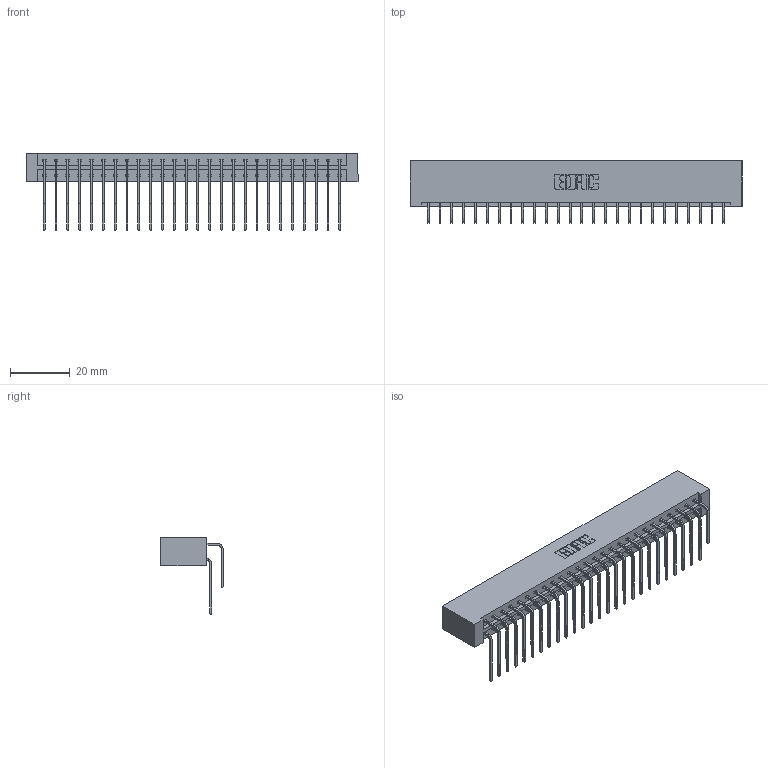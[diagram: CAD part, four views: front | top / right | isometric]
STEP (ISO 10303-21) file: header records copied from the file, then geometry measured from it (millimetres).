
FILE_DESCRIPTION (( 'STEP AP203' ), '1' );
FILE_NAME ('833-052-559-201.STEP', '2020-06-04T19:59:02', ( '' ), ( '' ), 'SwSTEP 2.0', 'SolidWorks 2020', '' );
FILE_SCHEMA (( 'CONFIG_CONTROL_DESIGN' ));
Length unit declared in the file: inch
Products named in the file (4): 833 Part_Lugless; 345-292-001_558 559 Tail - 1; 345-292-001_559 Tail - 2; 833-052-559-201
Assembly tree (53 placements, depth 2):
  833-052-559-201
    833 Part_Lugless
    345-292-001_558 559 Tail - 1  x26
    345-292-001_559 Tail - 2  x26
Bounding box: 111.28 x 20.9 x 25.53 mm (x, y, z)
Volume: 12143.4 mm3; surface area: 15703.1 mm2
Topology: 53 solids, 53 shells, 2914 faces, 8659 edges, 5702 vertices
Faces by surface type: plane 2042, cylinder 872
Entity records: 20303 total; most frequent: CARTESIAN_POINT 3433, ORIENTED_EDGE 3318, DIRECTION 2935, EDGE_CURVE 1659, LINE 1499, VECTOR 1499, VERTEX_POINT 1102, AXIS2_PLACEMENT_3D 718
